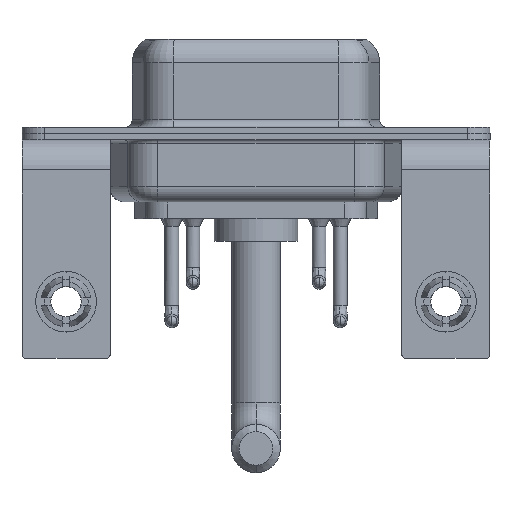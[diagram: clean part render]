
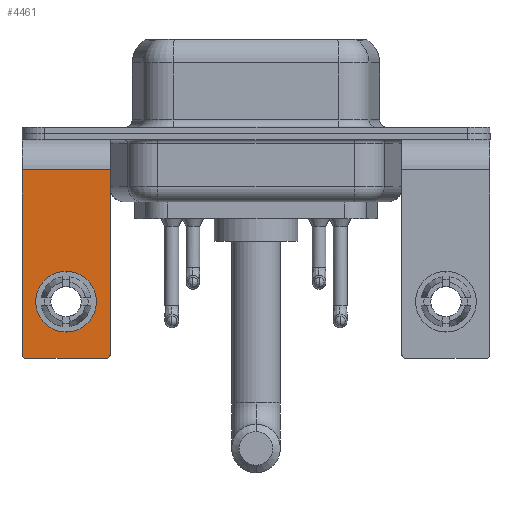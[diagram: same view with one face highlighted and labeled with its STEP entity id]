
A CAD part, front view. The second image highlights one B-rep face of the part: STEP entity #4461.
In plain terms, the highlighted planar face has unit normal (0, -1, 0).
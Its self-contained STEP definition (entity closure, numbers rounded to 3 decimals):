
#42 = CARTESIAN_POINT ( 'NONE',  ( 0., -6.25, -11.07 ) ) ;
#215 = EDGE_CURVE ( 'NONE', #7030, #7543, #2822, .T. ) ;
#513 = EDGE_CURVE ( 'NONE', #11707, #4549, #14274, .T. ) ;
#906 = EDGE_CURVE ( 'NONE', #7030, #2578, #11272, .T. ) ;
#1527 = EDGE_CURVE ( 'NONE', #17743, #14475, #2666, .T. ) ;
#1787 = CARTESIAN_POINT ( 'NONE',  ( 0., -6.25, -9.07 ) ) ;
#2298 = CARTESIAN_POINT ( 'NONE',  ( -2.9, -6.25, -2.4 ) ) ;
#2578 = VERTEX_POINT ( 'NONE', #5833 ) ;
#2666 = LINE ( 'NONE', #16772, #11602 ) ;
#2713 = DIRECTION ( 'NONE',  ( 0., 0., 1. ) ) ;
#2822 = LINE ( 'NONE', #10291, #4000 ) ;
#3064 = EDGE_CURVE ( 'NONE', #4549, #11707, #4057, .T. ) ;
#3141 = DIRECTION ( 'NONE',  ( 0., 1., 0. ) ) ;
#3373 = LINE ( 'NONE', #4615, #9263 ) ;
#3474 = CARTESIAN_POINT ( 'NONE',  ( 2.65, -6.25, -14.55 ) ) ;
#4000 = VECTOR ( 'NONE', #10201, 1000. ) ;
#4057 = CIRCLE ( 'NONE', #10093, 2. ) ;
#4461 = ADVANCED_FACE ( 'NONE', ( #15593, #18605 ), #9992, .F. ) ;
#4549 = VERTEX_POINT ( 'NONE', #1787 ) ;
#4615 = CARTESIAN_POINT ( 'NONE',  ( -2.9, -6.25, -2.4 ) ) ;
#4809 = DIRECTION ( 'NONE',  ( 0., 0., 1. ) ) ;
#5194 = CARTESIAN_POINT ( 'NONE',  ( 0., -6.25, -11.07 ) ) ;
#5197 = ORIENTED_EDGE ( 'NONE', *, *, #3064, .T. ) ;
#5283 = ORIENTED_EDGE ( 'NONE', *, *, #906, .T. ) ;
#5568 = VERTEX_POINT ( 'NONE', #13333 ) ;
#5572 = EDGE_LOOP ( 'NONE', ( #14969, #5197 ) ) ;
#5602 = AXIS2_PLACEMENT_3D ( 'NONE', #15765, #8574, #2713 ) ;
#5833 = CARTESIAN_POINT ( 'NONE',  ( 2.9, -6.25, -14.55 ) ) ;
#6121 = AXIS2_PLACEMENT_3D ( 'NONE', #5194, #9632, #9713 ) ;
#6414 = CARTESIAN_POINT ( 'NONE',  ( 0., -6.25, -13.07 ) ) ;
#6610 = ORIENTED_EDGE ( 'NONE', *, *, #15189, .T. ) ;
#6732 = LINE ( 'NONE', #17214, #11801 ) ;
#7030 = VERTEX_POINT ( 'NONE', #11477 ) ;
#7543 = VERTEX_POINT ( 'NONE', #8234 ) ;
#7598 = EDGE_CURVE ( 'NONE', #17743, #2578, #6732, .T. ) ;
#7655 = AXIS2_PLACEMENT_3D ( 'NONE', #3474, #7721, #4809 ) ;
#7721 = DIRECTION ( 'NONE',  ( 0., -1., 0. ) ) ;
#8234 = CARTESIAN_POINT ( 'NONE',  ( -2.65, -6.25, -14.8 ) ) ;
#8574 = DIRECTION ( 'NONE',  ( 0., 1., 0. ) ) ;
#8762 = DIRECTION ( 'NONE',  ( 0., 0., -1. ) ) ;
#8806 = DIRECTION ( 'NONE',  ( 0., 0., 1. ) ) ;
#9263 = VECTOR ( 'NONE', #8762, 1000. ) ;
#9632 = DIRECTION ( 'NONE',  ( 0., 1., 0. ) ) ;
#9713 = DIRECTION ( 'NONE',  ( 0., 0., 1. ) ) ;
#9761 = DIRECTION ( 'NONE',  ( 0., 0., 1. ) ) ;
#9992 = PLANE ( 'NONE',  #5602 ) ;
#10093 = AXIS2_PLACEMENT_3D ( 'NONE', #42, #3141, #8806 ) ;
#10201 = DIRECTION ( 'NONE',  ( -1., 0., 0. ) ) ;
#10291 = CARTESIAN_POINT ( 'NONE',  ( 2.9, -6.25, -14.8 ) ) ;
#11272 = CIRCLE ( 'NONE', #7655, 0.25 ) ;
#11347 = ORIENTED_EDGE ( 'NONE', *, *, #7598, .F. ) ;
#11477 = CARTESIAN_POINT ( 'NONE',  ( 2.65, -6.25, -14.8 ) ) ;
#11602 = VECTOR ( 'NONE', #15462, 1000. ) ;
#11707 = VERTEX_POINT ( 'NONE', #6414 ) ;
#11801 = VECTOR ( 'NONE', #14204, 1000. ) ;
#12551 = CIRCLE ( 'NONE', #14081, 0.25 ) ;
#12774 = ORIENTED_EDGE ( 'NONE', *, *, #14080, .T. ) ;
#13333 = CARTESIAN_POINT ( 'NONE',  ( -2.9, -6.25, -14.55 ) ) ;
#13697 = ORIENTED_EDGE ( 'NONE', *, *, #1527, .T. ) ;
#14080 = EDGE_CURVE ( 'NONE', #5568, #7543, #12551, .T. ) ;
#14081 = AXIS2_PLACEMENT_3D ( 'NONE', #15463, #18102, #9761 ) ;
#14204 = DIRECTION ( 'NONE',  ( 0., 0., -1. ) ) ;
#14274 = CIRCLE ( 'NONE', #6121, 2. ) ;
#14475 = VERTEX_POINT ( 'NONE', #2298 ) ;
#14969 = ORIENTED_EDGE ( 'NONE', *, *, #513, .T. ) ;
#14988 = CARTESIAN_POINT ( 'NONE',  ( 2.9, -6.25, -2.4 ) ) ;
#15189 = EDGE_CURVE ( 'NONE', #14475, #5568, #3373, .T. ) ;
#15462 = DIRECTION ( 'NONE',  ( -1., 0., 0. ) ) ;
#15463 = CARTESIAN_POINT ( 'NONE',  ( -2.65, -6.25, -14.55 ) ) ;
#15593 = FACE_BOUND ( 'NONE', #5572, .T. ) ;
#15765 = CARTESIAN_POINT ( 'NONE',  ( 2.9, -6.25, -2.4 ) ) ;
#16772 = CARTESIAN_POINT ( 'NONE',  ( 2.9, -6.25, -2.4 ) ) ;
#17214 = CARTESIAN_POINT ( 'NONE',  ( 2.9, -6.25, -2.4 ) ) ;
#17516 = ORIENTED_EDGE ( 'NONE', *, *, #215, .F. ) ;
#17743 = VERTEX_POINT ( 'NONE', #14988 ) ;
#18102 = DIRECTION ( 'NONE',  ( 0., -1., 0. ) ) ;
#18317 = EDGE_LOOP ( 'NONE', ( #6610, #12774, #17516, #5283, #11347, #13697 ) ) ;
#18605 = FACE_OUTER_BOUND ( 'NONE', #18317, .T. ) ;
